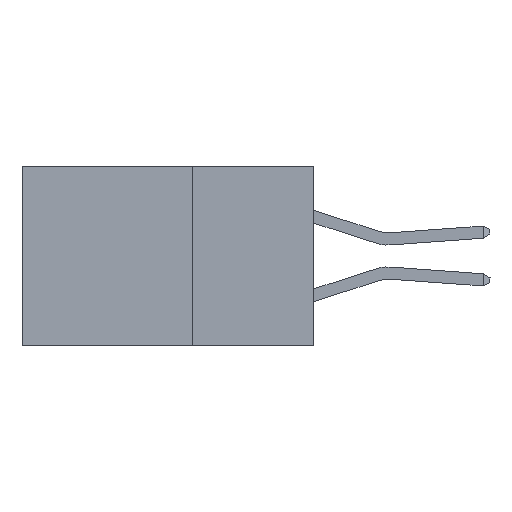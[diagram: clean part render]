
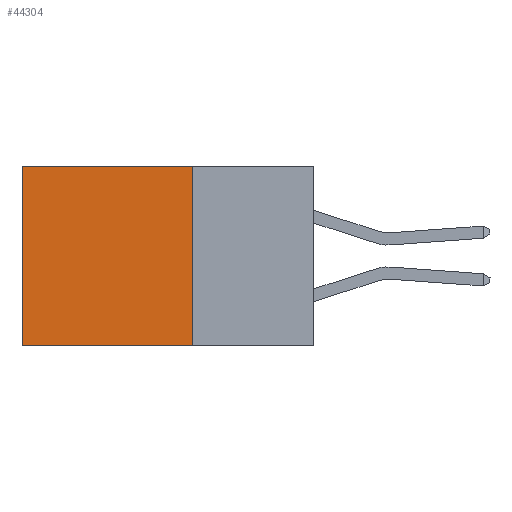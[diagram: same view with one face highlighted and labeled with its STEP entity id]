
A CAD part, left-side view. The second image highlights one B-rep face of the part: STEP entity #44304.
In plain terms, the highlighted planar face has unit normal (-1, 0, 0).
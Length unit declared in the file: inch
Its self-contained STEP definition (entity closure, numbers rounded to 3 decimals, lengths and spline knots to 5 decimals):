
#157 = LINE ( 'NONE', #26516, #9364 ) ;
#4086 = LINE ( 'NONE', #5204, #11671 ) ;
#5204 = CARTESIAN_POINT ( 'NONE',  ( 0.2875, 0.25, -0.37 ) ) ;
#5353 = DIRECTION ( 'NONE',  ( 0., 1., 0. ) ) ;
#7667 = DIRECTION ( 'NONE',  ( 0., 1., 0. ) ) ;
#8549 = VERTEX_POINT ( 'NONE', #14855 ) ;
#9364 = VECTOR ( 'NONE', #33757, 39.37008 ) ;
#10012 = ORIENTED_EDGE ( 'NONE', *, *, #30838, .T. ) ;
#11342 = VECTOR ( 'NONE', #22195, 39.37008 ) ;
#11671 = VECTOR ( 'NONE', #5353, 39.37008 ) ;
#12820 = EDGE_CURVE ( 'NONE', #8549, #40972, #24895, .T. ) ;
#13265 = PLANE ( 'NONE',  #15344 ) ;
#13566 = DIRECTION ( 'NONE',  ( 0., 0., -1. ) ) ;
#14368 = CARTESIAN_POINT ( 'NONE',  ( 0.2875, 0.6, -0.37 ) ) ;
#14855 = CARTESIAN_POINT ( 'NONE',  ( 0.2875, 0.25, 0. ) ) ;
#15344 = AXIS2_PLACEMENT_3D ( 'NONE', #20825, #37716, #13566 ) ;
#18565 = EDGE_LOOP ( 'NONE', ( #35186, #43635, #24062, #10012 ) ) ;
#20825 = CARTESIAN_POINT ( 'NONE',  ( 0.2875, 0.25, 0. ) ) ;
#22195 = DIRECTION ( 'NONE',  ( 0., 0., -1. ) ) ;
#24062 = ORIENTED_EDGE ( 'NONE', *, *, #12820, .F. ) ;
#24723 = CARTESIAN_POINT ( 'NONE',  ( 0.2875, 0.25, 0. ) ) ;
#24895 = LINE ( 'NONE', #43025, #11342 ) ;
#26516 = CARTESIAN_POINT ( 'NONE',  ( 0.2875, 0.6, 0. ) ) ;
#28877 = EDGE_CURVE ( 'NONE', #37885, #43753, #157, .T. ) ;
#30838 = EDGE_CURVE ( 'NONE', #8549, #37885, #35622, .T. ) ;
#32455 = EDGE_CURVE ( 'NONE', #40972, #43753, #4086, .T. ) ;
#33757 = DIRECTION ( 'NONE',  ( 0., 0., -1. ) ) ;
#35186 = ORIENTED_EDGE ( 'NONE', *, *, #28877, .T. ) ;
#35622 = LINE ( 'NONE', #24723, #36191 ) ;
#36191 = VECTOR ( 'NONE', #7667, 39.37008 ) ;
#36394 = CARTESIAN_POINT ( 'NONE',  ( 0.2875, 0.25, -0.37 ) ) ;
#37716 = DIRECTION ( 'NONE',  ( 1., 0., 0. ) ) ;
#37885 = VERTEX_POINT ( 'NONE', #39877 ) ;
#39877 = CARTESIAN_POINT ( 'NONE',  ( 0.2875, 0.6, 0. ) ) ;
#40575 = FACE_OUTER_BOUND ( 'NONE', #18565, .T. ) ;
#40972 = VERTEX_POINT ( 'NONE', #36394 ) ;
#43025 = CARTESIAN_POINT ( 'NONE',  ( 0.2875, 0.25, 0. ) ) ;
#43635 = ORIENTED_EDGE ( 'NONE', *, *, #32455, .F. ) ;
#43753 = VERTEX_POINT ( 'NONE', #14368 ) ;
#44304 = ADVANCED_FACE ( 'NONE', ( #40575 ), #13265, .F. ) ;
